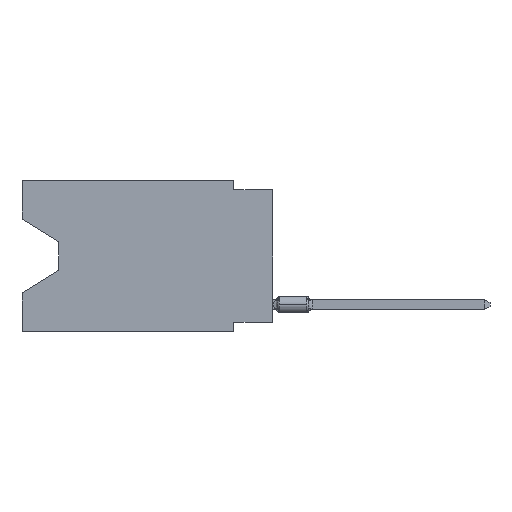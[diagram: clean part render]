
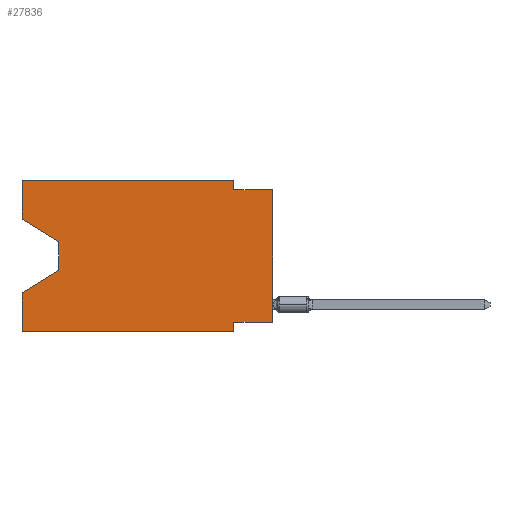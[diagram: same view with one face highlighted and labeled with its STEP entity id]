
A CAD part, left-side view. The second image highlights one B-rep face of the part: STEP entity #27836.
In plain terms, the highlighted planar face has unit normal (-1, 0, 0).
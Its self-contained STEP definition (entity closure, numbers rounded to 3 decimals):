
#118 = CARTESIAN_POINT ( 'NONE',  ( 0., 0., -0.635 ) ) ;
#827 = ORIENTED_EDGE ( 'NONE', *, *, #1796, .F. ) ;
#1717 = CARTESIAN_POINT ( 'NONE',  ( 0., 0., -0.635 ) ) ;
#1743 = LINE ( 'NONE', #14698, #19881 ) ;
#1796 = EDGE_CURVE ( 'NONE', #9172, #17178, #15246, .T. ) ;
#3055 = ORIENTED_EDGE ( 'NONE', *, *, #9298, .F. ) ;
#3185 = DIRECTION ( 'NONE',  ( 0., 0., 1. ) ) ;
#3380 = VECTOR ( 'NONE', #17179, 1000. ) ;
#3575 = EDGE_CURVE ( 'NONE', #11578, #14401, #24842, .T. ) ;
#3780 = DIRECTION ( 'NONE',  ( 0., 0., -1. ) ) ;
#3782 = LINE ( 'NONE', #26767, #26679 ) ;
#4112 = VECTOR ( 'NONE', #8653, 1000. ) ;
#4337 = ORIENTED_EDGE ( 'NONE', *, *, #13838, .F. ) ;
#4575 = DIRECTION ( 'NONE',  ( 1., 0., 0. ) ) ;
#5239 = EDGE_LOOP ( 'NONE', ( #11190, #18912, #20288, #6554, #17716, #26981, #10642, #26326, #3055, #827, #4337, #14423 ) ) ;
#5640 = EDGE_CURVE ( 'NONE', #22172, #16303, #27041, .T. ) ;
#5951 = EDGE_CURVE ( 'NONE', #23688, #6838, #7984, .T. ) ;
#6554 = ORIENTED_EDGE ( 'NONE', *, *, #5951, .F. ) ;
#6626 = CARTESIAN_POINT ( 'NONE',  ( 0., 16.383, 0. ) ) ;
#6838 = VERTEX_POINT ( 'NONE', #9683 ) ;
#6917 = CARTESIAN_POINT ( 'NONE',  ( 0., 2.54, 0. ) ) ;
#7563 = CARTESIAN_POINT ( 'NONE',  ( 0., 16.383, 0. ) ) ;
#7720 = CARTESIAN_POINT ( 'NONE',  ( 0., 2.54, -9.906 ) ) ;
#7984 = LINE ( 'NONE', #7563, #13627 ) ;
#8303 = LINE ( 'NONE', #23258, #12629 ) ;
#8446 = LINE ( 'NONE', #118, #3380 ) ;
#8632 = VERTEX_POINT ( 'NONE', #15272 ) ;
#8653 = DIRECTION ( 'NONE',  ( 0., 0.855, -0.519 ) ) ;
#9172 = VERTEX_POINT ( 'NONE', #22423 ) ;
#9298 = EDGE_CURVE ( 'NONE', #17178, #27198, #8446, .T. ) ;
#9683 = CARTESIAN_POINT ( 'NONE',  ( 0., 16.383, -7.36 ) ) ;
#9891 = CARTESIAN_POINT ( 'NONE',  ( 0., 16.383, -2.546 ) ) ;
#10642 = ORIENTED_EDGE ( 'NONE', *, *, #25968, .F. ) ;
#11117 = DIRECTION ( 'NONE',  ( 0., 0., 1. ) ) ;
#11142 = LINE ( 'NONE', #23551, #16309 ) ;
#11190 = ORIENTED_EDGE ( 'NONE', *, *, #3575, .T. ) ;
#11542 = VERTEX_POINT ( 'NONE', #16866 ) ;
#11578 = VERTEX_POINT ( 'NONE', #20805 ) ;
#11917 = CARTESIAN_POINT ( 'NONE',  ( 0., 16.383, -9.906 ) ) ;
#12353 = CARTESIAN_POINT ( 'NONE',  ( 0., 2.54, -9.271 ) ) ;
#12445 = CARTESIAN_POINT ( 'NONE',  ( 0., 0., -9.271 ) ) ;
#12629 = VECTOR ( 'NONE', #21009, 1000. ) ;
#13138 = VECTOR ( 'NONE', #11117, 1000. ) ;
#13155 = CARTESIAN_POINT ( 'NONE',  ( 0., 13.97, -5.893 ) ) ;
#13169 = DIRECTION ( 'NONE',  ( 0., 0., -1. ) ) ;
#13298 = CARTESIAN_POINT ( 'NONE',  ( 0., 13.97, -4.013 ) ) ;
#13438 = LINE ( 'NONE', #17955, #20810 ) ;
#13574 = FACE_OUTER_BOUND ( 'NONE', #5239, .T. ) ;
#13627 = VECTOR ( 'NONE', #3185, 1000. ) ;
#13838 = EDGE_CURVE ( 'NONE', #11542, #9172, #11142, .T. ) ;
#14401 = VERTEX_POINT ( 'NONE', #13298 ) ;
#14423 = ORIENTED_EDGE ( 'NONE', *, *, #15152, .F. ) ;
#14517 = CARTESIAN_POINT ( 'NONE',  ( 0., 2.54, -9.906 ) ) ;
#14531 = VECTOR ( 'NONE', #3780, 1000. ) ;
#14628 = EDGE_CURVE ( 'NONE', #14401, #8632, #1743, .T. ) ;
#14698 = CARTESIAN_POINT ( 'NONE',  ( 0., 13.97, -4.013 ) ) ;
#15152 = EDGE_CURVE ( 'NONE', #11578, #11542, #26352, .T. ) ;
#15237 = DIRECTION ( 'NONE',  ( 0., -1., 0. ) ) ;
#15246 = LINE ( 'NONE', #6917, #23696 ) ;
#15272 = CARTESIAN_POINT ( 'NONE',  ( 0., 13.97, -5.893 ) ) ;
#15294 = PLANE ( 'NONE',  #24134 ) ;
#15627 = EDGE_CURVE ( 'NONE', #15935, #27198, #13438, .T. ) ;
#15935 = VERTEX_POINT ( 'NONE', #12445 ) ;
#16303 = VERTEX_POINT ( 'NONE', #14517 ) ;
#16309 = VECTOR ( 'NONE', #15237, 1000. ) ;
#16804 = DIRECTION ( 'NONE',  ( 0., -0.855, -0.519 ) ) ;
#16866 = CARTESIAN_POINT ( 'NONE',  ( 0., 16.383, 0. ) ) ;
#17178 = VERTEX_POINT ( 'NONE', #19524 ) ;
#17179 = DIRECTION ( 'NONE',  ( 0., -1., 0. ) ) ;
#17231 = DIRECTION ( 'NONE',  ( 0., 0., -1. ) ) ;
#17716 = ORIENTED_EDGE ( 'NONE', *, *, #18585, .T. ) ;
#17955 = CARTESIAN_POINT ( 'NONE',  ( 0., 0., 0. ) ) ;
#18585 = EDGE_CURVE ( 'NONE', #23688, #16303, #8303, .T. ) ;
#18912 = ORIENTED_EDGE ( 'NONE', *, *, #14628, .T. ) ;
#18943 = VECTOR ( 'NONE', #16804, 1000. ) ;
#19065 = EDGE_CURVE ( 'NONE', #8632, #6838, #27843, .T. ) ;
#19524 = CARTESIAN_POINT ( 'NONE',  ( 0., 2.54, -0.635 ) ) ;
#19881 = VECTOR ( 'NONE', #17231, 1000. ) ;
#20271 = DIRECTION ( 'NONE',  ( 0., 1., 0. ) ) ;
#20288 = ORIENTED_EDGE ( 'NONE', *, *, #19065, .T. ) ;
#20805 = CARTESIAN_POINT ( 'NONE',  ( 0., 16.383, -2.546 ) ) ;
#20810 = VECTOR ( 'NONE', #22039, 1000. ) ;
#21009 = DIRECTION ( 'NONE',  ( 0., -1., 0. ) ) ;
#21869 = DIRECTION ( 'NONE',  ( 0., 0., -1. ) ) ;
#22039 = DIRECTION ( 'NONE',  ( 0., 0., 1. ) ) ;
#22172 = VERTEX_POINT ( 'NONE', #12353 ) ;
#22423 = CARTESIAN_POINT ( 'NONE',  ( 0., 2.54, 0. ) ) ;
#23258 = CARTESIAN_POINT ( 'NONE',  ( 0., 16.383, -9.906 ) ) ;
#23551 = CARTESIAN_POINT ( 'NONE',  ( 0., 16.383, 0. ) ) ;
#23688 = VERTEX_POINT ( 'NONE', #11917 ) ;
#23696 = VECTOR ( 'NONE', #21869, 1000. ) ;
#23885 = CARTESIAN_POINT ( 'NONE',  ( 0., 16.383, 0. ) ) ;
#24134 = AXIS2_PLACEMENT_3D ( 'NONE', #23885, #4575, #13169 ) ;
#24842 = LINE ( 'NONE', #9891, #18943 ) ;
#25968 = EDGE_CURVE ( 'NONE', #15935, #22172, #3782, .T. ) ;
#26326 = ORIENTED_EDGE ( 'NONE', *, *, #15627, .T. ) ;
#26352 = LINE ( 'NONE', #6626, #13138 ) ;
#26679 = VECTOR ( 'NONE', #20271, 1000. ) ;
#26767 = CARTESIAN_POINT ( 'NONE',  ( 0., 0., -9.271 ) ) ;
#26981 = ORIENTED_EDGE ( 'NONE', *, *, #5640, .F. ) ;
#27041 = LINE ( 'NONE', #7720, #14531 ) ;
#27198 = VERTEX_POINT ( 'NONE', #1717 ) ;
#27836 = ADVANCED_FACE ( 'NONE', ( #13574 ), #15294, .F. ) ;
#27843 = LINE ( 'NONE', #13155, #4112 ) ;
